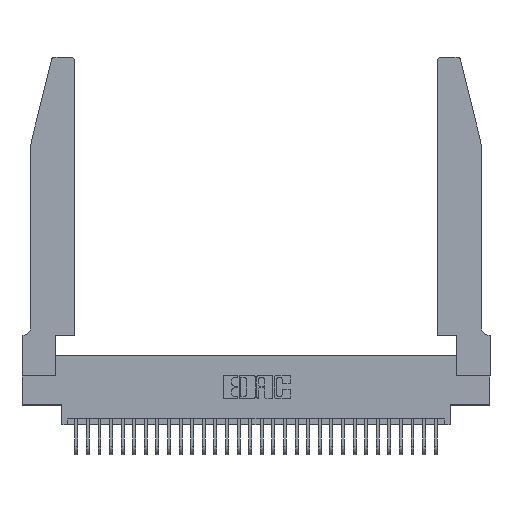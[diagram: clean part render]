
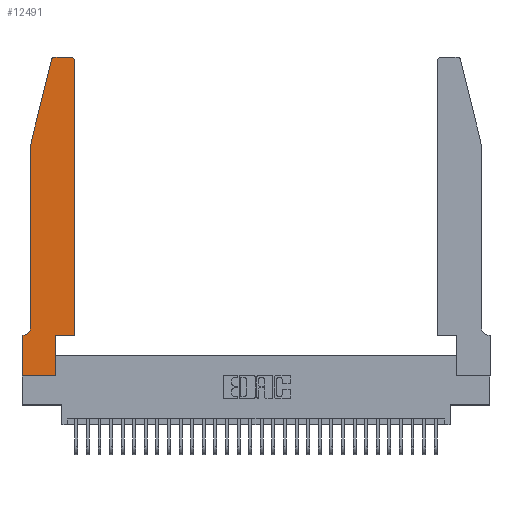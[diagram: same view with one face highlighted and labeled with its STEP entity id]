
A CAD part, top view. The second image highlights one B-rep face of the part: STEP entity #12491.
In plain terms, the highlighted planar face has unit normal (0, 0, 1).
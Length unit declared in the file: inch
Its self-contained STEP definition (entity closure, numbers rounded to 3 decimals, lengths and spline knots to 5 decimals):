
#133 = EDGE_CURVE ( 'NONE', #29983, #4061, #4710, .T. ) ;
#353 = CARTESIAN_POINT ( 'NONE',  ( 0.0055, 0.35, 0.37 ) ) ;
#829 = AXIS2_PLACEMENT_3D ( 'NONE', #30803, #10466, #20914 ) ;
#2684 = CARTESIAN_POINT ( 'NONE',  ( 0., 0., 0.37 ) ) ;
#2840 = AXIS2_PLACEMENT_3D ( 'NONE', #16787, #19442, #24696 ) ;
#3348 = LINE ( 'NONE', #19577, #21292 ) ;
#3998 = ORIENTED_EDGE ( 'NONE', *, *, #23158, .T. ) ;
#4061 = VERTEX_POINT ( 'NONE', #20022 ) ;
#4513 = CARTESIAN_POINT ( 'NONE',  ( 0.0755, 2., 0.37 ) ) ;
#4710 = LINE ( 'NONE', #2684, #10341 ) ;
#4841 = VERTEX_POINT ( 'NONE', #16880 ) ;
#5347 = VERTEX_POINT ( 'NONE', #11523 ) ;
#6129 = CARTESIAN_POINT ( 'NONE',  ( 0.4505, 0.35, 0.37 ) ) ;
#6831 = CIRCLE ( 'NONE', #2840, 0.03 ) ;
#7649 = LINE ( 'NONE', #27100, #15210 ) ;
#7745 = LINE ( 'NONE', #25791, #15697 ) ;
#8482 = ORIENTED_EDGE ( 'NONE', *, *, #16122, .T. ) ;
#8691 = CIRCLE ( 'NONE', #22187, 0.03 ) ;
#8988 = VECTOR ( 'NONE', #21453, 39.37008 ) ;
#9153 = VERTEX_POINT ( 'NONE', #25394 ) ;
#9582 = LINE ( 'NONE', #21147, #15148 ) ;
#10341 = VECTOR ( 'NONE', #23865, 39.37008 ) ;
#10466 = DIRECTION ( 'NONE',  ( 0., 0., -1. ) ) ;
#10621 = VECTOR ( 'NONE', #14091, 39.37008 ) ;
#11523 = CARTESIAN_POINT ( 'NONE',  ( 0.2865, 0.35, 0.37 ) ) ;
#11874 = LINE ( 'NONE', #31876, #10621 ) ;
#12491 = ADVANCED_FACE ( 'NONE', ( #16071 ), #18497, .T. ) ;
#12893 = LINE ( 'NONE', #6129, #21230 ) ;
#13388 = ORIENTED_EDGE ( 'NONE', *, *, #29751, .T. ) ;
#14091 = DIRECTION ( 'NONE',  ( -1., 0., 0. ) ) ;
#14575 = DIRECTION ( 'NONE',  ( 0., -1., 0. ) ) ;
#14741 = VERTEX_POINT ( 'NONE', #353 ) ;
#14838 = ORIENTED_EDGE ( 'NONE', *, *, #28240, .T. ) ;
#14999 = CARTESIAN_POINT ( 'NONE',  ( 0.2865, 0., 0.37 ) ) ;
#15148 = VECTOR ( 'NONE', #28586, 39.37008 ) ;
#15210 = VECTOR ( 'NONE', #32345, 39.37008 ) ;
#15280 = EDGE_CURVE ( 'NONE', #20667, #4841, #8691, .T. ) ;
#15644 = VERTEX_POINT ( 'NONE', #26508 ) ;
#15697 = VECTOR ( 'NONE', #18134, 39.37008 ) ;
#15842 = ORIENTED_EDGE ( 'NONE', *, *, #30611, .T. ) ;
#16071 = FACE_OUTER_BOUND ( 'NONE', #27125, .T. ) ;
#16122 = EDGE_CURVE ( 'NONE', #9153, #14741, #23390, .T. ) ;
#16147 = DIRECTION ( 'NONE',  ( 0., 1., 0. ) ) ;
#16156 = DIRECTION ( 'NONE',  ( 0., 0., 1. ) ) ;
#16787 = CARTESIAN_POINT ( 'NONE',  ( 0.4205, 2.72, 0.37 ) ) ;
#16880 = CARTESIAN_POINT ( 'NONE',  ( 0.25487, 2.72718, 0.37 ) ) ;
#17021 = EDGE_CURVE ( 'NONE', #14741, #29983, #11874, .T. ) ;
#17025 = ORIENTED_EDGE ( 'NONE', *, *, #29687, .T. ) ;
#17601 = EDGE_CURVE ( 'NONE', #5347, #29388, #18162, .T. ) ;
#17653 = DIRECTION ( 'NONE',  ( 1., 0., 0. ) ) ;
#18112 = CARTESIAN_POINT ( 'NONE',  ( 0.4505, 2.72, 0.37 ) ) ;
#18134 = DIRECTION ( 'NONE',  ( -1., 0., 0. ) ) ;
#18162 = LINE ( 'NONE', #28764, #8988 ) ;
#18497 = PLANE ( 'NONE',  #21048 ) ;
#19121 = ORIENTED_EDGE ( 'NONE', *, *, #15280, .T. ) ;
#19442 = DIRECTION ( 'NONE',  ( 0., 0., 1. ) ) ;
#19577 = CARTESIAN_POINT ( 'NONE',  ( 0.0755, 2., 0.37 ) ) ;
#20022 = CARTESIAN_POINT ( 'NONE',  ( 0., 0., 0.37 ) ) ;
#20425 = CARTESIAN_POINT ( 'NONE',  ( 0., 0.35, 0.37 ) ) ;
#20667 = VERTEX_POINT ( 'NONE', #22616 ) ;
#20914 = DIRECTION ( 'NONE',  ( -1., 0., 0. ) ) ;
#21039 = DIRECTION ( 'NONE',  ( 1., 0., 0. ) ) ;
#21048 = AXIS2_PLACEMENT_3D ( 'NONE', #21257, #16156, #21039 ) ;
#21147 = CARTESIAN_POINT ( 'NONE',  ( 0., 0., 0.37 ) ) ;
#21230 = VECTOR ( 'NONE', #31409, 39.37008 ) ;
#21257 = CARTESIAN_POINT ( 'NONE',  ( 0., 0.35, 0.37 ) ) ;
#21292 = VECTOR ( 'NONE', #14575, 39.37008 ) ;
#21453 = DIRECTION ( 'NONE',  ( 1., 0., 0. ) ) ;
#22187 = AXIS2_PLACEMENT_3D ( 'NONE', #30527, #30420, #17653 ) ;
#22616 = CARTESIAN_POINT ( 'NONE',  ( 0.284, 2.75, 0.37 ) ) ;
#23158 = EDGE_CURVE ( 'NONE', #28623, #9153, #3348, .T. ) ;
#23390 = CIRCLE ( 'NONE', #829, 0.07 ) ;
#23739 = VERTEX_POINT ( 'NONE', #14999 ) ;
#23865 = DIRECTION ( 'NONE',  ( 0., -1., 0. ) ) ;
#23942 = CARTESIAN_POINT ( 'NONE',  ( 0.2865, 0.35, 0.37 ) ) ;
#24083 = EDGE_CURVE ( 'NONE', #29388, #32463, #12893, .T. ) ;
#24696 = DIRECTION ( 'NONE',  ( 1., 0., 0. ) ) ;
#25375 = LINE ( 'NONE', #23942, #30921 ) ;
#25394 = CARTESIAN_POINT ( 'NONE',  ( 0.0755, 0.42, 0.37 ) ) ;
#25786 = ORIENTED_EDGE ( 'NONE', *, *, #25845, .T. ) ;
#25791 = CARTESIAN_POINT ( 'NONE',  ( 0.2605, 2.75, 0.37 ) ) ;
#25845 = EDGE_CURVE ( 'NONE', #23739, #5347, #25375, .T. ) ;
#26508 = CARTESIAN_POINT ( 'NONE',  ( 0.4205, 2.75, 0.37 ) ) ;
#27100 = CARTESIAN_POINT ( 'NONE',  ( 0.0755, 2., 0.37 ) ) ;
#27125 = EDGE_LOOP ( 'NONE', ( #14838, #19121, #13388, #3998, #8482, #27429, #29395, #15842, #25786, #28362, #27787, #17025 ) ) ;
#27429 = ORIENTED_EDGE ( 'NONE', *, *, #17021, .T. ) ;
#27787 = ORIENTED_EDGE ( 'NONE', *, *, #24083, .T. ) ;
#28004 = CARTESIAN_POINT ( 'NONE',  ( 0.4505, 0.35, 0.37 ) ) ;
#28240 = EDGE_CURVE ( 'NONE', #15644, #20667, #7745, .T. ) ;
#28362 = ORIENTED_EDGE ( 'NONE', *, *, #17601, .T. ) ;
#28586 = DIRECTION ( 'NONE',  ( 1., 0., 0. ) ) ;
#28623 = VERTEX_POINT ( 'NONE', #4513 ) ;
#28764 = CARTESIAN_POINT ( 'NONE',  ( 0.4505, 0.35, 0.37 ) ) ;
#29388 = VERTEX_POINT ( 'NONE', #28004 ) ;
#29395 = ORIENTED_EDGE ( 'NONE', *, *, #133, .T. ) ;
#29687 = EDGE_CURVE ( 'NONE', #32463, #15644, #6831, .T. ) ;
#29751 = EDGE_CURVE ( 'NONE', #4841, #28623, #7649, .T. ) ;
#29983 = VERTEX_POINT ( 'NONE', #20425 ) ;
#30420 = DIRECTION ( 'NONE',  ( 0., 0., 1. ) ) ;
#30527 = CARTESIAN_POINT ( 'NONE',  ( 0.284, 2.72, 0.37 ) ) ;
#30611 = EDGE_CURVE ( 'NONE', #4061, #23739, #9582, .T. ) ;
#30803 = CARTESIAN_POINT ( 'NONE',  ( 0.0055, 0.42, 0.37 ) ) ;
#30921 = VECTOR ( 'NONE', #16147, 39.37008 ) ;
#31409 = DIRECTION ( 'NONE',  ( 0., 1., 0. ) ) ;
#31876 = CARTESIAN_POINT ( 'NONE',  ( 0.0755, 0.35, 0.37 ) ) ;
#32345 = DIRECTION ( 'NONE',  ( -0.239, -0.971, 0. ) ) ;
#32463 = VERTEX_POINT ( 'NONE', #18112 ) ;
